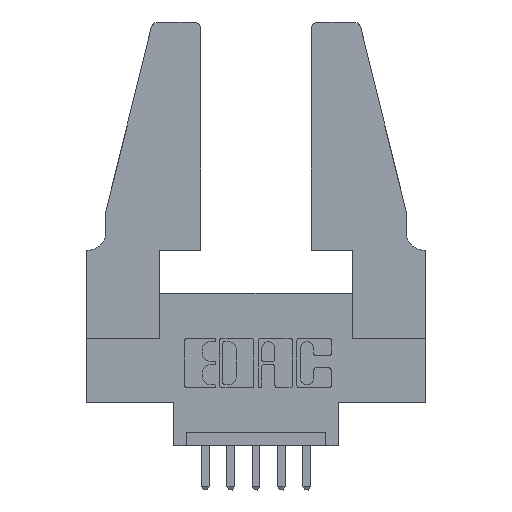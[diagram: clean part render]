
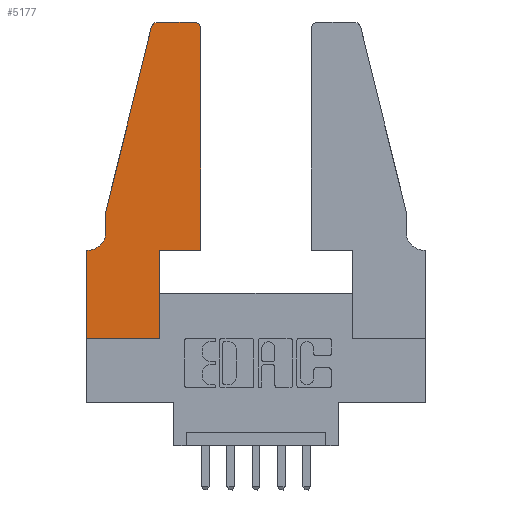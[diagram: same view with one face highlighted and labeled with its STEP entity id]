
A CAD part, top view. The second image highlights one B-rep face of the part: STEP entity #5177.
In plain terms, the highlighted planar face has unit normal (0, 0, 1).
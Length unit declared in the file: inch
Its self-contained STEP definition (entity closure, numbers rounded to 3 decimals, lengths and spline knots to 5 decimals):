
#49 = ORIENTED_EDGE ( 'NONE', *, *, #7924, .T. ) ;
#385 = CARTESIAN_POINT ( 'NONE',  ( 0.0755, 0.5, 0.37 ) ) ;
#548 = CIRCLE ( 'NONE', #6878, 0.07 ) ;
#600 = CARTESIAN_POINT ( 'NONE',  ( 0.284, 1.25, 0.37 ) ) ;
#634 = ORIENTED_EDGE ( 'NONE', *, *, #1062, .T. ) ;
#659 = CARTESIAN_POINT ( 'NONE',  ( 0., 0., 0.37 ) ) ;
#766 = ORIENTED_EDGE ( 'NONE', *, *, #3462, .T. ) ;
#849 = DIRECTION ( 'NONE',  ( 0., 0., 1. ) ) ;
#1062 = EDGE_CURVE ( 'NONE', #7103, #8273, #10955, .T. ) ;
#1071 = ORIENTED_EDGE ( 'NONE', *, *, #6567, .T. ) ;
#1097 = LINE ( 'NONE', #3568, #10028 ) ;
#1211 = AXIS2_PLACEMENT_3D ( 'NONE', #8638, #849, #4210 ) ;
#1322 = CARTESIAN_POINT ( 'NONE',  ( 0.0055, 0.42, 0.37 ) ) ;
#1402 = CARTESIAN_POINT ( 'NONE',  ( 0.25487, 1.22718, 0.37 ) ) ;
#1626 = VERTEX_POINT ( 'NONE', #2830 ) ;
#1677 = CIRCLE ( 'NONE', #2020, 0.03 ) ;
#1800 = DIRECTION ( 'NONE',  ( 0., -1., 0. ) ) ;
#1915 = VECTOR ( 'NONE', #3742, 39.37008 ) ;
#2020 = AXIS2_PLACEMENT_3D ( 'NONE', #2080, #7221, #6267 ) ;
#2048 = CARTESIAN_POINT ( 'NONE',  ( 0.0755, 0.42, 0.37 ) ) ;
#2080 = CARTESIAN_POINT ( 'NONE',  ( 0.4205, 1.22, 0.37 ) ) ;
#2285 = AXIS2_PLACEMENT_3D ( 'NONE', #7270, #5586, #7344 ) ;
#2537 = LINE ( 'NONE', #659, #4138 ) ;
#2550 = CARTESIAN_POINT ( 'NONE',  ( 0., 0.35, 0.37 ) ) ;
#2619 = CARTESIAN_POINT ( 'NONE',  ( 0.0755, 0.5, 0.37 ) ) ;
#2658 = CARTESIAN_POINT ( 'NONE',  ( 0., 0., 0.37 ) ) ;
#2689 = VERTEX_POINT ( 'NONE', #3097 ) ;
#2708 = CARTESIAN_POINT ( 'NONE',  ( 0.0755, 0.5, 0.37 ) ) ;
#2801 = VECTOR ( 'NONE', #5402, 39.37008 ) ;
#2830 = CARTESIAN_POINT ( 'NONE',  ( 0.4505, 1.22, 0.37 ) ) ;
#2894 = ORIENTED_EDGE ( 'NONE', *, *, #3401, .T. ) ;
#3097 = CARTESIAN_POINT ( 'NONE',  ( 0.4205, 1.25, 0.37 ) ) ;
#3274 = CIRCLE ( 'NONE', #2285, 0.03 ) ;
#3401 = EDGE_CURVE ( 'NONE', #3724, #11064, #4837, .T. ) ;
#3462 = EDGE_CURVE ( 'NONE', #8273, #8458, #1097, .T. ) ;
#3490 = CARTESIAN_POINT ( 'NONE',  ( 0.2865, 0.35, 0.37 ) ) ;
#3568 = CARTESIAN_POINT ( 'NONE',  ( 0.4505, 0.35, 0.37 ) ) ;
#3724 = VERTEX_POINT ( 'NONE', #1402 ) ;
#3736 = ORIENTED_EDGE ( 'NONE', *, *, #5096, .T. ) ;
#3742 = DIRECTION ( 'NONE',  ( 0., 1., 0. ) ) ;
#3759 = LINE ( 'NONE', #2708, #5782 ) ;
#3768 = EDGE_CURVE ( 'NONE', #6946, #9464, #10273, .T. ) ;
#4138 = VECTOR ( 'NONE', #8416, 39.37008 ) ;
#4153 = VECTOR ( 'NONE', #10116, 39.37008 ) ;
#4210 = DIRECTION ( 'NONE',  ( 1., 0., 0. ) ) ;
#4473 = EDGE_CURVE ( 'NONE', #8458, #1626, #9752, .T. ) ;
#4491 = VERTEX_POINT ( 'NONE', #600 ) ;
#4595 = ORIENTED_EDGE ( 'NONE', *, *, #4473, .T. ) ;
#4837 = LINE ( 'NONE', #2619, #7447 ) ;
#4938 = LINE ( 'NONE', #8905, #8095 ) ;
#5096 = EDGE_CURVE ( 'NONE', #10781, #7103, #2537, .T. ) ;
#5121 = EDGE_LOOP ( 'NONE', ( #7769, #7194, #2894, #49, #9301, #6279, #10309, #3736, #634, #766, #4595, #1071 ) ) ;
#5172 = DIRECTION ( 'NONE',  ( 1., 0., 0. ) ) ;
#5177 = ADVANCED_FACE ( 'NONE', ( #9988 ), #11093, .T. ) ;
#5287 = DIRECTION ( 'NONE',  ( -0.239, -0.971, 0. ) ) ;
#5402 = DIRECTION ( 'NONE',  ( 0., -1., 0. ) ) ;
#5586 = DIRECTION ( 'NONE',  ( 0., 0., 1. ) ) ;
#5782 = VECTOR ( 'NONE', #1800, 39.37008 ) ;
#5836 = DIRECTION ( 'NONE',  ( 0., 1., 0. ) ) ;
#5990 = CARTESIAN_POINT ( 'NONE',  ( 0., 0., 0.37 ) ) ;
#6143 = EDGE_CURVE ( 'NONE', #4491, #3724, #3274, .T. ) ;
#6267 = DIRECTION ( 'NONE',  ( 1., 0., 0. ) ) ;
#6279 = ORIENTED_EDGE ( 'NONE', *, *, #3768, .T. ) ;
#6504 = VERTEX_POINT ( 'NONE', #2048 ) ;
#6567 = EDGE_CURVE ( 'NONE', #1626, #2689, #1677, .T. ) ;
#6855 = CARTESIAN_POINT ( 'NONE',  ( 0.4505, 0.35, 0.37 ) ) ;
#6878 = AXIS2_PLACEMENT_3D ( 'NONE', #1322, #9856, #10789 ) ;
#6946 = VERTEX_POINT ( 'NONE', #8637 ) ;
#7103 = VERTEX_POINT ( 'NONE', #9215 ) ;
#7194 = ORIENTED_EDGE ( 'NONE', *, *, #6143, .T. ) ;
#7221 = DIRECTION ( 'NONE',  ( 0., 0., 1. ) ) ;
#7270 = CARTESIAN_POINT ( 'NONE',  ( 0.284, 1.22, 0.37 ) ) ;
#7344 = DIRECTION ( 'NONE',  ( 1., 0., 0. ) ) ;
#7443 = VECTOR ( 'NONE', #5836, 39.37008 ) ;
#7447 = VECTOR ( 'NONE', #5287, 39.37008 ) ;
#7465 = CARTESIAN_POINT ( 'NONE',  ( 0.0755, 0.35, 0.37 ) ) ;
#7566 = CARTESIAN_POINT ( 'NONE',  ( 0.4505, 0.35, 0.37 ) ) ;
#7769 = ORIENTED_EDGE ( 'NONE', *, *, #9593, .T. ) ;
#7924 = EDGE_CURVE ( 'NONE', #11064, #6504, #3759, .T. ) ;
#8095 = VECTOR ( 'NONE', #9900, 39.37008 ) ;
#8273 = VERTEX_POINT ( 'NONE', #9302 ) ;
#8416 = DIRECTION ( 'NONE',  ( 1., 0., 0. ) ) ;
#8458 = VERTEX_POINT ( 'NONE', #6855 ) ;
#8564 = EDGE_CURVE ( 'NONE', #9464, #10781, #9064, .T. ) ;
#8637 = CARTESIAN_POINT ( 'NONE',  ( 0.0055, 0.35, 0.37 ) ) ;
#8638 = CARTESIAN_POINT ( 'NONE',  ( 0., 0.35, 0.37 ) ) ;
#8700 = EDGE_CURVE ( 'NONE', #6504, #6946, #548, .T. ) ;
#8905 = CARTESIAN_POINT ( 'NONE',  ( 0.2605, 1.25, 0.37 ) ) ;
#9064 = LINE ( 'NONE', #2658, #2801 ) ;
#9215 = CARTESIAN_POINT ( 'NONE',  ( 0.2865, 0., 0.37 ) ) ;
#9301 = ORIENTED_EDGE ( 'NONE', *, *, #8700, .T. ) ;
#9302 = CARTESIAN_POINT ( 'NONE',  ( 0.2865, 0.35, 0.37 ) ) ;
#9464 = VERTEX_POINT ( 'NONE', #2550 ) ;
#9593 = EDGE_CURVE ( 'NONE', #2689, #4491, #4938, .T. ) ;
#9752 = LINE ( 'NONE', #7566, #7443 ) ;
#9856 = DIRECTION ( 'NONE',  ( 0., 0., -1. ) ) ;
#9900 = DIRECTION ( 'NONE',  ( -1., 0., 0. ) ) ;
#9988 = FACE_OUTER_BOUND ( 'NONE', #5121, .T. ) ;
#10028 = VECTOR ( 'NONE', #5172, 39.37008 ) ;
#10116 = DIRECTION ( 'NONE',  ( -1., 0., 0. ) ) ;
#10273 = LINE ( 'NONE', #7465, #4153 ) ;
#10309 = ORIENTED_EDGE ( 'NONE', *, *, #8564, .T. ) ;
#10781 = VERTEX_POINT ( 'NONE', #5990 ) ;
#10789 = DIRECTION ( 'NONE',  ( -1., 0., 0. ) ) ;
#10955 = LINE ( 'NONE', #3490, #1915 ) ;
#11064 = VERTEX_POINT ( 'NONE', #385 ) ;
#11093 = PLANE ( 'NONE',  #1211 ) ;
